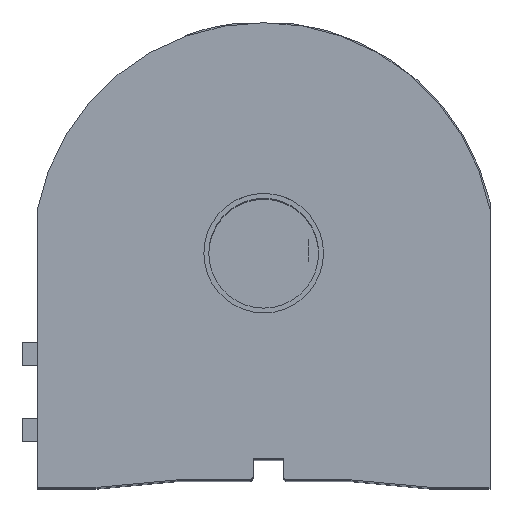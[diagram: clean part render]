
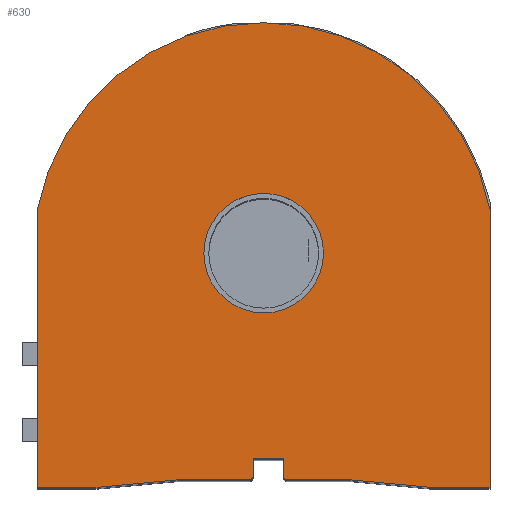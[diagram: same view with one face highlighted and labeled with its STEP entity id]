
A CAD part, top view. The second image highlights one B-rep face of the part: STEP entity #630.
In plain terms, the highlighted planar face has unit normal (0, 0, 1).
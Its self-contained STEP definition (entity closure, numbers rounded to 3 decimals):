
#1 = DIRECTION ( 'NONE',  ( 1., 0., 0. ) ) ;
#30 = CARTESIAN_POINT ( 'NONE',  ( 6.083, -59., 80. ) ) ;
#43 = VERTEX_POINT ( 'NONE', #2899 ) ;
#53 = CARTESIAN_POINT ( 'NONE',  ( 43.909, -61., 80. ) ) ;
#105 = VECTOR ( 'NONE', #2277, 1000. ) ;
#118 = LINE ( 'NONE', #200, #1092 ) ;
#168 = LINE ( 'NONE', #3421, #105 ) ;
#182 = ORIENTED_EDGE ( 'NONE', *, *, #1059, .F. ) ;
#200 = CARTESIAN_POINT ( 'NONE',  ( -43.909, -61., 80. ) ) ;
#205 = VERTEX_POINT ( 'NONE', #30 ) ;
#248 = VERTEX_POINT ( 'NONE', #1450 ) ;
#272 = ORIENTED_EDGE ( 'NONE', *, *, #4875, .T. ) ;
#366 = DIRECTION ( 'NONE',  ( -1., 0., 0. ) ) ;
#380 = LINE ( 'NONE', #3690, #5231 ) ;
#441 = LINE ( 'NONE', #2336, #2057 ) ;
#473 = DIRECTION ( 'NONE',  ( 0., 0., -1. ) ) ;
#577 = ORIENTED_EDGE ( 'NONE', *, *, #1986, .T. ) ;
#630 = ADVANCED_FACE ( 'NONE', ( #2958, #2041 ), #1730, .F. ) ;
#705 = EDGE_CURVE ( 'NONE', #1607, #205, #168, .T. ) ;
#743 = DIRECTION ( 'NONE',  ( 1., 0., 0. ) ) ;
#765 = CARTESIAN_POINT ( 'NONE',  ( -2.75, -53.5, 80. ) ) ;
#770 = LINE ( 'NONE', #797, #2060 ) ;
#797 = CARTESIAN_POINT ( 'NONE',  ( 22.5, -59., 80. ) ) ;
#823 = DIRECTION ( 'NONE',  ( 0., 1., 0. ) ) ;
#909 = VERTEX_POINT ( 'NONE', #1099 ) ;
#936 = VERTEX_POINT ( 'NONE', #2007 ) ;
#1059 = EDGE_CURVE ( 'NONE', #2175, #248, #2917, .T. ) ;
#1092 = VECTOR ( 'NONE', #1785, 1000. ) ;
#1099 = CARTESIAN_POINT ( 'NONE',  ( -22.5, -59., 80. ) ) ;
#1126 = VECTOR ( 'NONE', #2021, 1000. ) ;
#1202 = DIRECTION ( 'NONE',  ( 0., -1., 0. ) ) ;
#1227 = VECTOR ( 'NONE', #4936, 1000. ) ;
#1230 = CARTESIAN_POINT ( 'NONE',  ( -3.75, -59., 80. ) ) ;
#1318 = DIRECTION ( 'NONE',  ( -1., 0., 0. ) ) ;
#1413 = EDGE_CURVE ( 'NONE', #909, #5303, #118, .T. ) ;
#1420 = AXIS2_PLACEMENT_3D ( 'NONE', #2549, #473, #1318 ) ;
#1450 = CARTESIAN_POINT ( 'NONE',  ( 15.56, 0., 80. ) ) ;
#1496 = ORIENTED_EDGE ( 'NONE', *, *, #2878, .F. ) ;
#1571 = VECTOR ( 'NONE', #4550, 1000. ) ;
#1589 = EDGE_CURVE ( 'NONE', #2965, #5303, #441, .T. ) ;
#1600 = ORIENTED_EDGE ( 'NONE', *, *, #2328, .T. ) ;
#1607 = VERTEX_POINT ( 'NONE', #5039 ) ;
#1730 = PLANE ( 'NONE',  #1420 ) ;
#1735 = ORIENTED_EDGE ( 'NONE', *, *, #3912, .T. ) ;
#1736 = VERTEX_POINT ( 'NONE', #4244 ) ;
#1785 = DIRECTION ( 'NONE',  ( -0.996, -0.093, 0. ) ) ;
#1891 = CIRCLE ( 'NONE', #3288, 1. ) ;
#1952 = CARTESIAN_POINT ( 'NONE',  ( 0., 0., 80. ) ) ;
#1962 = ORIENTED_EDGE ( 'NONE', *, *, #1413, .F. ) ;
#1986 = EDGE_CURVE ( 'NONE', #2253, #936, #3211, .T. ) ;
#2006 = CARTESIAN_POINT ( 'NONE',  ( -43.909, -61., 80. ) ) ;
#2007 = CARTESIAN_POINT ( 'NONE',  ( -58.909, 11.39, 80. ) ) ;
#2021 = DIRECTION ( 'NONE',  ( -1., 0., 0. ) ) ;
#2035 = DIRECTION ( 'NONE',  ( 1., 0., 0. ) ) ;
#2041 = FACE_OUTER_BOUND ( 'NONE', #4177, .T. ) ;
#2048 = ORIENTED_EDGE ( 'NONE', *, *, #3561, .F. ) ;
#2057 = VECTOR ( 'NONE', #1, 1000. ) ;
#2060 = VECTOR ( 'NONE', #3643, 1000. ) ;
#2065 = DIRECTION ( 'NONE',  ( 0., 0., 1. ) ) ;
#2082 = LINE ( 'NONE', #3360, #1571 ) ;
#2125 = VERTEX_POINT ( 'NONE', #3356 ) ;
#2156 = CIRCLE ( 'NONE', #4868, 15.56 ) ;
#2175 = VERTEX_POINT ( 'NONE', #3544 ) ;
#2177 = VERTEX_POINT ( 'NONE', #2746 ) ;
#2236 = ORIENTED_EDGE ( 'NONE', *, *, #1589, .T. ) ;
#2253 = VERTEX_POINT ( 'NONE', #3189 ) ;
#2258 = DIRECTION ( 'NONE',  ( -1., 0., 0. ) ) ;
#2277 = DIRECTION ( 'NONE',  ( -1., 0., 0. ) ) ;
#2304 = LINE ( 'NONE', #2333, #3716 ) ;
#2328 = EDGE_CURVE ( 'NONE', #2177, #205, #3236, .T. ) ;
#2333 = CARTESIAN_POINT ( 'NONE',  ( -58.909, -61., 80. ) ) ;
#2336 = CARTESIAN_POINT ( 'NONE',  ( 58.909, -61., 80. ) ) ;
#2424 = CARTESIAN_POINT ( 'NONE',  ( 5.083, -53.5, 80. ) ) ;
#2468 = LINE ( 'NONE', #4087, #2841 ) ;
#2493 = VECTOR ( 'NONE', #823, 1000. ) ;
#2543 = CARTESIAN_POINT ( 'NONE',  ( 0., 0., 80. ) ) ;
#2549 = CARTESIAN_POINT ( 'NONE',  ( 0., 0., 80. ) ) ;
#2579 = ORIENTED_EDGE ( 'NONE', *, *, #3845, .F. ) ;
#2666 = CARTESIAN_POINT ( 'NONE',  ( -58.909, -61., 80. ) ) ;
#2675 = AXIS2_PLACEMENT_3D ( 'NONE', #3773, #4601, #2813 ) ;
#2701 = EDGE_CURVE ( 'NONE', #5417, #1607, #3669, .T. ) ;
#2746 = CARTESIAN_POINT ( 'NONE',  ( 5.083, -58., 80. ) ) ;
#2813 = DIRECTION ( 'NONE',  ( -1., 0., 0. ) ) ;
#2815 = CARTESIAN_POINT ( 'NONE',  ( 43.909, -61., 80. ) ) ;
#2841 = VECTOR ( 'NONE', #743, 1000. ) ;
#2855 = LINE ( 'NONE', #2424, #1126 ) ;
#2878 = EDGE_CURVE ( 'NONE', #2177, #43, #2082, .T. ) ;
#2899 = CARTESIAN_POINT ( 'NONE',  ( 5.083, -53.5, 80. ) ) ;
#2917 = CIRCLE ( 'NONE', #4323, 15.56 ) ;
#2958 = FACE_BOUND ( 'NONE', #3129, .T. ) ;
#2965 = VERTEX_POINT ( 'NONE', #2666 ) ;
#3129 = EDGE_LOOP ( 'NONE', ( #3772, #182 ) ) ;
#3184 = ORIENTED_EDGE ( 'NONE', *, *, #3694, .T. ) ;
#3189 = CARTESIAN_POINT ( 'NONE',  ( 58.909, 11.39, 80. ) ) ;
#3197 = ORIENTED_EDGE ( 'NONE', *, *, #2701, .F. ) ;
#3211 = CIRCLE ( 'NONE', #2675, 60. ) ;
#3236 = CIRCLE ( 'NONE', #5343, 1. ) ;
#3241 = VERTEX_POINT ( 'NONE', #1230 ) ;
#3252 = ORIENTED_EDGE ( 'NONE', *, *, #3299, .F. ) ;
#3288 = AXIS2_PLACEMENT_3D ( 'NONE', #4121, #2065, #366 ) ;
#3299 = EDGE_CURVE ( 'NONE', #4064, #1736, #380, .T. ) ;
#3336 = DIRECTION ( 'NONE',  ( 0., 0., 1. ) ) ;
#3356 = CARTESIAN_POINT ( 'NONE',  ( 58.909, -61., 80. ) ) ;
#3360 = CARTESIAN_POINT ( 'NONE',  ( 5.083, -66.165, 80. ) ) ;
#3421 = CARTESIAN_POINT ( 'NONE',  ( 22.5, -59., 80. ) ) ;
#3544 = CARTESIAN_POINT ( 'NONE',  ( -15.56, 0., 80. ) ) ;
#3561 = EDGE_CURVE ( 'NONE', #43, #4064, #2855, .T. ) ;
#3615 = DIRECTION ( 'NONE',  ( 0., 0., 1. ) ) ;
#3643 = DIRECTION ( 'NONE',  ( -1., 0., 0. ) ) ;
#3669 = LINE ( 'NONE', #2815, #1227 ) ;
#3690 = CARTESIAN_POINT ( 'NONE',  ( -2.75, -53.5, 80. ) ) ;
#3694 = EDGE_CURVE ( 'NONE', #936, #2965, #2304, .T. ) ;
#3702 = CARTESIAN_POINT ( 'NONE',  ( 58.909, -61., 80. ) ) ;
#3716 = VECTOR ( 'NONE', #5175, 1000. ) ;
#3772 = ORIENTED_EDGE ( 'NONE', *, *, #4758, .F. ) ;
#3773 = CARTESIAN_POINT ( 'NONE',  ( 0., 0., 80. ) ) ;
#3803 = EDGE_CURVE ( 'NONE', #5417, #2125, #2468, .T. ) ;
#3845 = EDGE_CURVE ( 'NONE', #3241, #909, #770, .T. ) ;
#3912 = EDGE_CURVE ( 'NONE', #2125, #2253, #5015, .T. ) ;
#3980 = CARTESIAN_POINT ( 'NONE',  ( 6.083, -58., 80. ) ) ;
#4064 = VERTEX_POINT ( 'NONE', #765 ) ;
#4073 = ORIENTED_EDGE ( 'NONE', *, *, #3803, .T. ) ;
#4087 = CARTESIAN_POINT ( 'NONE',  ( 58.909, -61., 80. ) ) ;
#4121 = CARTESIAN_POINT ( 'NONE',  ( -3.75, -58., 80. ) ) ;
#4177 = EDGE_LOOP ( 'NONE', ( #1496, #1600, #4261, #3197, #4073, #1735, #577, #3184, #2236, #1962, #2579, #272, #3252, #2048 ) ) ;
#4244 = CARTESIAN_POINT ( 'NONE',  ( -2.75, -58., 80. ) ) ;
#4261 = ORIENTED_EDGE ( 'NONE', *, *, #705, .F. ) ;
#4323 = AXIS2_PLACEMENT_3D ( 'NONE', #2543, #3336, #2035 ) ;
#4391 = DIRECTION ( 'NONE',  ( 0., 0., 1. ) ) ;
#4550 = DIRECTION ( 'NONE',  ( 0., 1., 0. ) ) ;
#4601 = DIRECTION ( 'NONE',  ( 0., 0., 1. ) ) ;
#4758 = EDGE_CURVE ( 'NONE', #248, #2175, #2156, .T. ) ;
#4868 = AXIS2_PLACEMENT_3D ( 'NONE', #1952, #3615, #5208 ) ;
#4875 = EDGE_CURVE ( 'NONE', #3241, #1736, #1891, .T. ) ;
#4936 = DIRECTION ( 'NONE',  ( -0.996, 0.093, 0. ) ) ;
#5015 = LINE ( 'NONE', #3702, #2493 ) ;
#5039 = CARTESIAN_POINT ( 'NONE',  ( 22.5, -59., 80. ) ) ;
#5175 = DIRECTION ( 'NONE',  ( 0., -1., 0. ) ) ;
#5208 = DIRECTION ( 'NONE',  ( 1., 0., 0. ) ) ;
#5231 = VECTOR ( 'NONE', #1202, 1000. ) ;
#5303 = VERTEX_POINT ( 'NONE', #2006 ) ;
#5343 = AXIS2_PLACEMENT_3D ( 'NONE', #3980, #4391, #2258 ) ;
#5417 = VERTEX_POINT ( 'NONE', #53 ) ;
